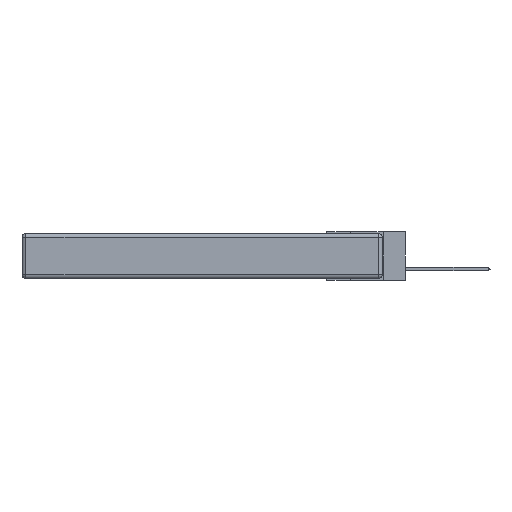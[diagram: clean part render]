
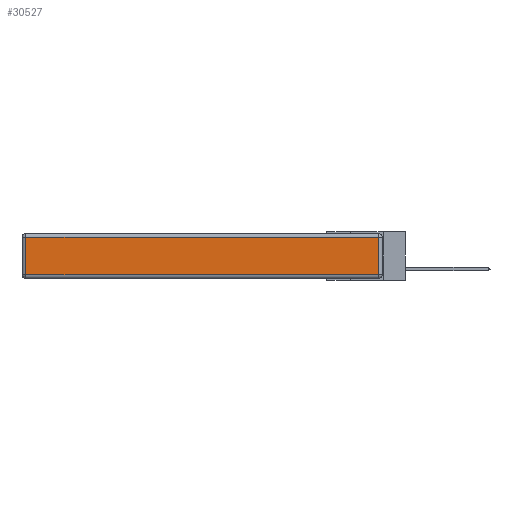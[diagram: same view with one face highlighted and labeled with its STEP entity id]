
A CAD part, left-side view. The second image highlights one B-rep face of the part: STEP entity #30527.
In plain terms, the highlighted planar face has unit normal (-1, 0, 0).
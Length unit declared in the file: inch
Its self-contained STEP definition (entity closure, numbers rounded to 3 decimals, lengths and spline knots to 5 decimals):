
#521 = CARTESIAN_POINT ( 'NONE',  ( 0., 2.72, -0.03 ) ) ;
#707 = CARTESIAN_POINT ( 'NONE',  ( 0., 0., -0.343 ) ) ;
#1163 = CARTESIAN_POINT ( 'NONE',  ( 0., 0., -0.313 ) ) ;
#1784 = LINE ( 'NONE', #17385, #19026 ) ;
#1843 = CARTESIAN_POINT ( 'NONE',  ( 0., 0.03, -0.313 ) ) ;
#2484 = EDGE_LOOP ( 'NONE', ( #16925, #16035, #7526, #15378 ) ) ;
#3640 = VECTOR ( 'NONE', #11608, 39.37008 ) ;
#4974 = VERTEX_POINT ( 'NONE', #9014 ) ;
#5333 = DIRECTION ( 'NONE',  ( -1., 0., 0. ) ) ;
#6591 = LINE ( 'NONE', #8067, #12324 ) ;
#6791 = LINE ( 'NONE', #1163, #18256 ) ;
#7526 = ORIENTED_EDGE ( 'NONE', *, *, #20249, .T. ) ;
#8067 = CARTESIAN_POINT ( 'NONE',  ( 0., 2.75, -0.03 ) ) ;
#9014 = CARTESIAN_POINT ( 'NONE',  ( 0., 2.72, -0.313 ) ) ;
#11608 = DIRECTION ( 'NONE',  ( 0., 0., 1. ) ) ;
#11674 = LINE ( 'NONE', #21544, #3640 ) ;
#11827 = CARTESIAN_POINT ( 'NONE',  ( 0., 0.03, -0.03 ) ) ;
#12324 = VECTOR ( 'NONE', #28043, 39.37008 ) ;
#12710 = PLANE ( 'NONE',  #13025 ) ;
#12712 = EDGE_CURVE ( 'NONE', #4974, #14658, #6791, .T. ) ;
#13025 = AXIS2_PLACEMENT_3D ( 'NONE', #707, #5333, #29815 ) ;
#14658 = VERTEX_POINT ( 'NONE', #1843 ) ;
#14856 = VERTEX_POINT ( 'NONE', #11827 ) ;
#15163 = EDGE_CURVE ( 'NONE', #28339, #4974, #1784, .T. ) ;
#15378 = ORIENTED_EDGE ( 'NONE', *, *, #15163, .T. ) ;
#16035 = ORIENTED_EDGE ( 'NONE', *, *, #16233, .T. ) ;
#16233 = EDGE_CURVE ( 'NONE', #14658, #14856, #11674, .T. ) ;
#16925 = ORIENTED_EDGE ( 'NONE', *, *, #12712, .T. ) ;
#17385 = CARTESIAN_POINT ( 'NONE',  ( 0., 2.72, -0.343 ) ) ;
#18256 = VECTOR ( 'NONE', #25867, 39.37008 ) ;
#19026 = VECTOR ( 'NONE', #19622, 39.37008 ) ;
#19622 = DIRECTION ( 'NONE',  ( 0., 0., -1. ) ) ;
#20249 = EDGE_CURVE ( 'NONE', #14856, #28339, #6591, .T. ) ;
#20776 = FACE_OUTER_BOUND ( 'NONE', #2484, .T. ) ;
#21544 = CARTESIAN_POINT ( 'NONE',  ( 0., 0.03, -0.343 ) ) ;
#25867 = DIRECTION ( 'NONE',  ( 0., -1., 0. ) ) ;
#28043 = DIRECTION ( 'NONE',  ( 0., 1., 0. ) ) ;
#28339 = VERTEX_POINT ( 'NONE', #521 ) ;
#29815 = DIRECTION ( 'NONE',  ( 0., 0., 1. ) ) ;
#30527 = ADVANCED_FACE ( 'NONE', ( #20776 ), #12710, .T. ) ;
